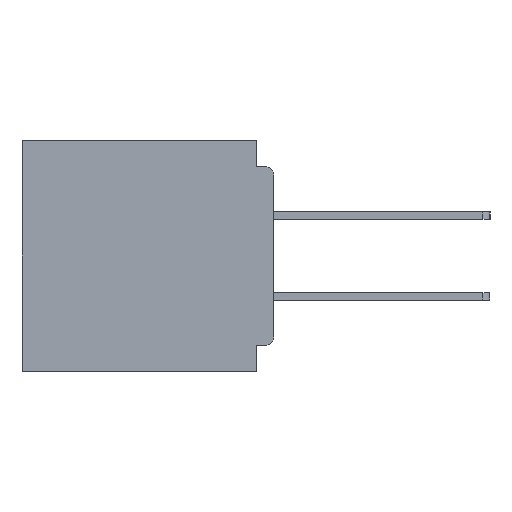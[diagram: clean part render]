
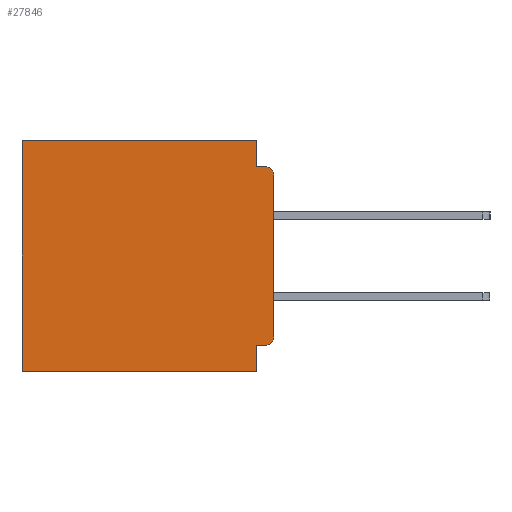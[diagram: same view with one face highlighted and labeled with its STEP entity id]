
A CAD part, left-side view. The second image highlights one B-rep face of the part: STEP entity #27846.
In plain terms, the highlighted planar face has unit normal (-1, 0, 0).
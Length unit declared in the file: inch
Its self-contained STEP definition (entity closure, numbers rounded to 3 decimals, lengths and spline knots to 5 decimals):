
#148 = CARTESIAN_POINT ( 'NONE',  ( 0.3, 0.015, -0.06 ) ) ;
#370 = CARTESIAN_POINT ( 'NONE',  ( 0.3, 0.437, 0. ) ) ;
#2222 = DIRECTION ( 'NONE',  ( -1., 0., 0. ) ) ;
#3084 = LINE ( 'NONE', #17756, #14117 ) ;
#3829 = ORIENTED_EDGE ( 'NONE', *, *, #47142, .T. ) ;
#3863 = VERTEX_POINT ( 'NONE', #21173 ) ;
#3965 = VERTEX_POINT ( 'NONE', #36801 ) ;
#4084 = DIRECTION ( 'NONE',  ( 0., 1., 0. ) ) ;
#4777 = CARTESIAN_POINT ( 'NONE',  ( 0.3, 0., -0.4 ) ) ;
#4827 = DIRECTION ( 'NONE',  ( 0., 0., -1. ) ) ;
#5121 = DIRECTION ( 'NONE',  ( 0., 0., -1. ) ) ;
#5340 = CARTESIAN_POINT ( 'NONE',  ( 0.3, 0.031, -0.4 ) ) ;
#6014 = DIRECTION ( 'NONE',  ( 0., 0., -1. ) ) ;
#6202 = VERTEX_POINT ( 'NONE', #58464 ) ;
#6446 = DIRECTION ( 'NONE',  ( 0., 0., -1. ) ) ;
#8129 = DIRECTION ( 'NONE',  ( 0., 1., 0. ) ) ;
#8219 = FACE_OUTER_BOUND ( 'NONE', #18675, .T. ) ;
#8409 = ORIENTED_EDGE ( 'NONE', *, *, #25496, .T. ) ;
#8430 = CARTESIAN_POINT ( 'NONE',  ( 0.3, 0.437, -0.4 ) ) ;
#9069 = EDGE_CURVE ( 'NONE', #32980, #31980, #3084, .T. ) ;
#9728 = LINE ( 'NONE', #8430, #31626 ) ;
#11045 = ORIENTED_EDGE ( 'NONE', *, *, #9069, .F. ) ;
#12975 = EDGE_CURVE ( 'NONE', #16356, #31980, #13580, .T. ) ;
#13580 = CIRCLE ( 'NONE', #41470, 0.015 ) ;
#14117 = VECTOR ( 'NONE', #59482, 39.37008 ) ;
#15694 = CARTESIAN_POINT ( 'NONE',  ( 0.3, 0.031, 0. ) ) ;
#15720 = VECTOR ( 'NONE', #6446, 39.37008 ) ;
#16356 = VERTEX_POINT ( 'NONE', #24507 ) ;
#17756 = CARTESIAN_POINT ( 'NONE',  ( 0.3, 0., -0.045 ) ) ;
#18298 = EDGE_CURVE ( 'NONE', #3863, #3965, #37959, .T. ) ;
#18468 = LINE ( 'NONE', #27446, #54051 ) ;
#18675 = EDGE_LOOP ( 'NONE', ( #52610, #22313, #11045, #22933, #3829, #35976, #39150, #58455, #46144, #8409 ) ) ;
#19287 = VERTEX_POINT ( 'NONE', #49854 ) ;
#19340 = LINE ( 'NONE', #43882, #28836 ) ;
#21173 = CARTESIAN_POINT ( 'NONE',  ( 0.3, 0.031, -0.355 ) ) ;
#21444 = EDGE_CURVE ( 'NONE', #55646, #32980, #41927, .T. ) ;
#22313 = ORIENTED_EDGE ( 'NONE', *, *, #12975, .T. ) ;
#22933 = ORIENTED_EDGE ( 'NONE', *, *, #21444, .F. ) ;
#24507 = CARTESIAN_POINT ( 'NONE',  ( 0.3, 0., -0.06 ) ) ;
#25496 = EDGE_CURVE ( 'NONE', #6202, #19287, #27447, .T. ) ;
#25932 = LINE ( 'NONE', #46203, #49155 ) ;
#27003 = DIRECTION ( 'NONE',  ( 0., 0., -1. ) ) ;
#27446 = CARTESIAN_POINT ( 'NONE',  ( 0.3, 0., -0.4 ) ) ;
#27447 = CIRCLE ( 'NONE', #48897, 0.015 ) ;
#27846 = ADVANCED_FACE ( 'NONE', ( #8219 ), #37628, .F. ) ;
#28836 = VECTOR ( 'NONE', #53194, 39.37008 ) ;
#30272 = CARTESIAN_POINT ( 'NONE',  ( 0.3, 0.015, -0.34 ) ) ;
#30326 = VECTOR ( 'NONE', #8129, 39.37008 ) ;
#31344 = CARTESIAN_POINT ( 'NONE',  ( 0.3, 0.437, -0.4 ) ) ;
#31626 = VECTOR ( 'NONE', #27003, 39.37008 ) ;
#31929 = AXIS2_PLACEMENT_3D ( 'NONE', #4777, #33977, #6014 ) ;
#31980 = VERTEX_POINT ( 'NONE', #56463 ) ;
#32844 = DIRECTION ( 'NONE',  ( -1., 0., 0. ) ) ;
#32980 = VERTEX_POINT ( 'NONE', #39362 ) ;
#33977 = DIRECTION ( 'NONE',  ( 1., 0., 0. ) ) ;
#34873 = DIRECTION ( 'NONE',  ( 0., 0., -1. ) ) ;
#35976 = ORIENTED_EDGE ( 'NONE', *, *, #55838, .T. ) ;
#36801 = CARTESIAN_POINT ( 'NONE',  ( 0.3, 0.031, -0.4 ) ) ;
#37628 = PLANE ( 'NONE',  #31929 ) ;
#37959 = LINE ( 'NONE', #5340, #48832 ) ;
#39150 = ORIENTED_EDGE ( 'NONE', *, *, #56025, .F. ) ;
#39362 = CARTESIAN_POINT ( 'NONE',  ( 0.3, 0.031, -0.045 ) ) ;
#40695 = CARTESIAN_POINT ( 'NONE',  ( 0.3, 0., -0.355 ) ) ;
#41042 = EDGE_CURVE ( 'NONE', #16356, #19287, #25932, .T. ) ;
#41470 = AXIS2_PLACEMENT_3D ( 'NONE', #148, #32844, #4827 ) ;
#41927 = LINE ( 'NONE', #15694, #15720 ) ;
#43882 = CARTESIAN_POINT ( 'NONE',  ( 0.3, 0., 0. ) ) ;
#44718 = LINE ( 'NONE', #40695, #30326 ) ;
#46144 = ORIENTED_EDGE ( 'NONE', *, *, #54634, .F. ) ;
#46203 = CARTESIAN_POINT ( 'NONE',  ( 0.3, 0., -0.4 ) ) ;
#47142 = EDGE_CURVE ( 'NONE', #55646, #51351, #19340, .T. ) ;
#48832 = VECTOR ( 'NONE', #5121, 39.37008 ) ;
#48897 = AXIS2_PLACEMENT_3D ( 'NONE', #30272, #2222, #34873 ) ;
#48911 = CARTESIAN_POINT ( 'NONE',  ( 0.3, 0.031, 0. ) ) ;
#49155 = VECTOR ( 'NONE', #50880, 39.37008 ) ;
#49854 = CARTESIAN_POINT ( 'NONE',  ( 0.3, 0., -0.34 ) ) ;
#50506 = VERTEX_POINT ( 'NONE', #31344 ) ;
#50880 = DIRECTION ( 'NONE',  ( 0., 0., -1. ) ) ;
#51351 = VERTEX_POINT ( 'NONE', #370 ) ;
#52610 = ORIENTED_EDGE ( 'NONE', *, *, #41042, .F. ) ;
#53194 = DIRECTION ( 'NONE',  ( 0., 1., 0. ) ) ;
#54051 = VECTOR ( 'NONE', #4084, 39.37008 ) ;
#54634 = EDGE_CURVE ( 'NONE', #6202, #3863, #44718, .T. ) ;
#55646 = VERTEX_POINT ( 'NONE', #48911 ) ;
#55838 = EDGE_CURVE ( 'NONE', #51351, #50506, #9728, .T. ) ;
#56025 = EDGE_CURVE ( 'NONE', #3965, #50506, #18468, .T. ) ;
#56463 = CARTESIAN_POINT ( 'NONE',  ( 0.3, 0.015, -0.045 ) ) ;
#58455 = ORIENTED_EDGE ( 'NONE', *, *, #18298, .F. ) ;
#58464 = CARTESIAN_POINT ( 'NONE',  ( 0.3, 0.015, -0.355 ) ) ;
#59482 = DIRECTION ( 'NONE',  ( 0., -1., 0. ) ) ;
